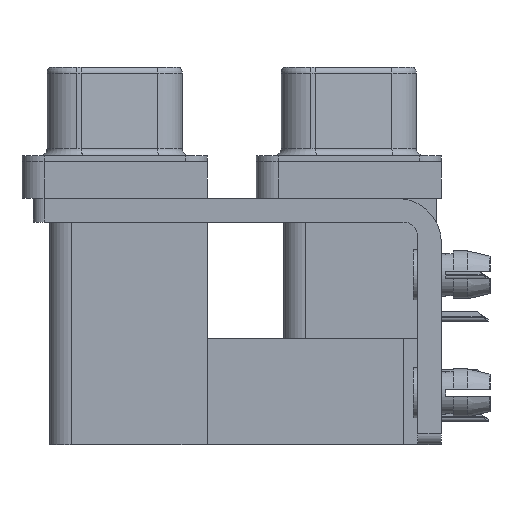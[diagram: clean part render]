
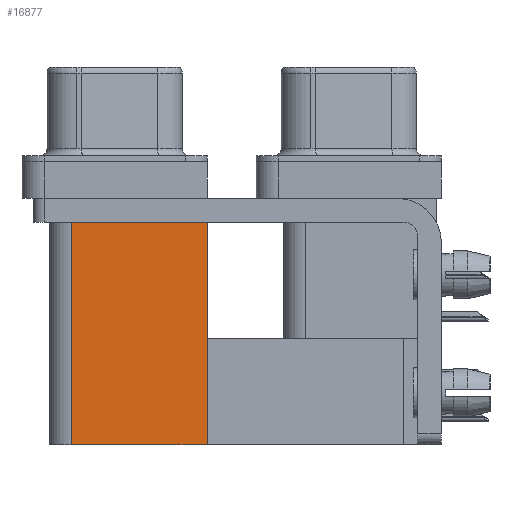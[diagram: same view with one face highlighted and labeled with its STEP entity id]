
A CAD part, left-side view. The second image highlights one B-rep face of the part: STEP entity #16877.
In plain terms, the highlighted planar face has unit normal (-1, 0, 0).
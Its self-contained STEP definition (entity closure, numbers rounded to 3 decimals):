
#529 = VERTEX_POINT ( 'NONE', #10899 ) ;
#685 = DIRECTION ( 'NONE',  ( 1., 0., 0. ) ) ;
#995 = AXIS2_PLACEMENT_3D ( 'NONE', #9710, #685, #18959 ) ;
#2984 = DIRECTION ( 'NONE',  ( 0., 0., 1. ) ) ;
#3500 = FACE_OUTER_BOUND ( 'NONE', #26663, .T. ) ;
#5799 = LINE ( 'NONE', #23864, #18873 ) ;
#6973 = DIRECTION ( 'NONE',  ( 0., 0., 1. ) ) ;
#7361 = CARTESIAN_POINT ( 'NONE',  ( 3.7, 9.6, -19.2 ) ) ;
#8374 = CARTESIAN_POINT ( 'NONE',  ( 3.7, 9.6, -19.2 ) ) ;
#8477 = CARTESIAN_POINT ( 'NONE',  ( 3.7, 18.8, -2.5 ) ) ;
#8515 = EDGE_CURVE ( 'NONE', #23384, #17135, #5799, .T. ) ;
#8533 = EDGE_CURVE ( 'NONE', #529, #17135, #9200, .T. ) ;
#9200 = LINE ( 'NONE', #21040, #13102 ) ;
#9710 = CARTESIAN_POINT ( 'NONE',  ( 3.7, 9.6, -19.2 ) ) ;
#10899 = CARTESIAN_POINT ( 'NONE',  ( 3.7, 18.8, -19.2 ) ) ;
#13102 = VECTOR ( 'NONE', #2984, 1000. ) ;
#15184 = DIRECTION ( 'NONE',  ( 0., 1., 0. ) ) ;
#16311 = EDGE_CURVE ( 'NONE', #30994, #529, #33050, .T. ) ;
#16877 = ADVANCED_FACE ( 'NONE', ( #3500 ), #27978, .F. ) ;
#17135 = VERTEX_POINT ( 'NONE', #8477 ) ;
#18237 = DIRECTION ( 'NONE',  ( 0., 1., 0. ) ) ;
#18807 = ORIENTED_EDGE ( 'NONE', *, *, #8533, .F. ) ;
#18873 = VECTOR ( 'NONE', #18237, 1000. ) ;
#18959 = DIRECTION ( 'NONE',  ( 0., 0., -1. ) ) ;
#21040 = CARTESIAN_POINT ( 'NONE',  ( 3.7, 18.8, -19.2 ) ) ;
#23384 = VERTEX_POINT ( 'NONE', #34921 ) ;
#23650 = ORIENTED_EDGE ( 'NONE', *, *, #39068, .T. ) ;
#23864 = CARTESIAN_POINT ( 'NONE',  ( 3.7, 9.6, -2.5 ) ) ;
#26663 = EDGE_LOOP ( 'NONE', ( #38172, #18807, #34256, #23650 ) ) ;
#27978 = PLANE ( 'NONE',  #995 ) ;
#30994 = VERTEX_POINT ( 'NONE', #35700 ) ;
#31432 = LINE ( 'NONE', #7361, #35218 ) ;
#32982 = VECTOR ( 'NONE', #15184, 1000. ) ;
#33050 = LINE ( 'NONE', #8374, #32982 ) ;
#34256 = ORIENTED_EDGE ( 'NONE', *, *, #16311, .F. ) ;
#34921 = CARTESIAN_POINT ( 'NONE',  ( 3.7, 9.6, -2.5 ) ) ;
#35218 = VECTOR ( 'NONE', #6973, 1000. ) ;
#35700 = CARTESIAN_POINT ( 'NONE',  ( 3.7, 9.6, -19.2 ) ) ;
#38172 = ORIENTED_EDGE ( 'NONE', *, *, #8515, .T. ) ;
#39068 = EDGE_CURVE ( 'NONE', #30994, #23384, #31432, .T. ) ;
